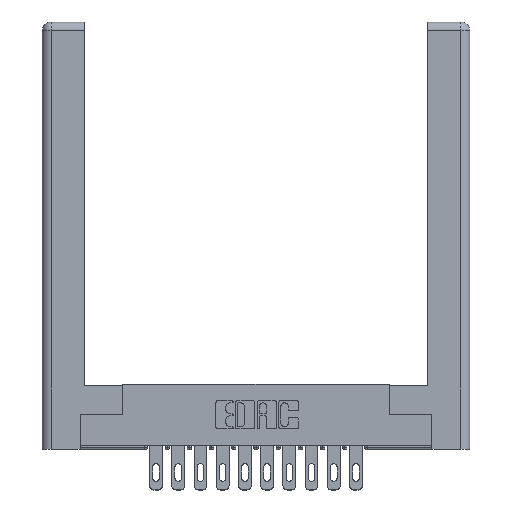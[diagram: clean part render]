
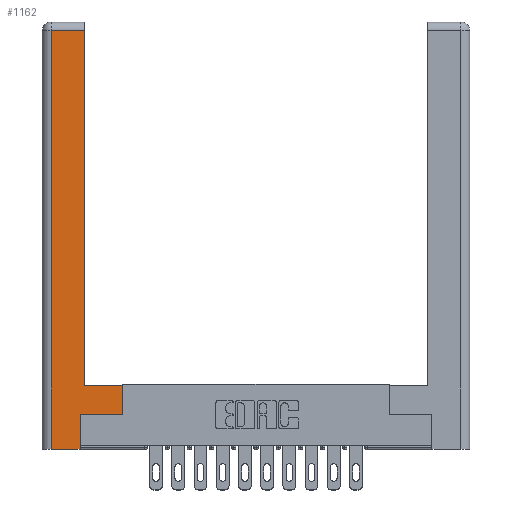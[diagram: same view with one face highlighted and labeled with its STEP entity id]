
A CAD part, top view. The second image highlights one B-rep face of the part: STEP entity #1162.
In plain terms, the highlighted planar face has unit normal (0, 0, 1).
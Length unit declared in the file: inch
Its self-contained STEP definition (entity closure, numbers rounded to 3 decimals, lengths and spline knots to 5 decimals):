
#121 = VERTEX_POINT ( 'NONE', #6297 ) ;
#192 = EDGE_CURVE ( 'NONE', #15788, #4579, #12210, .T. ) ;
#621 = DIRECTION ( 'NONE',  ( 0., 0., -1. ) ) ;
#874 = LINE ( 'NONE', #12211, #16828 ) ;
#901 = EDGE_CURVE ( 'NONE', #14083, #13963, #13010, .T. ) ;
#926 = VECTOR ( 'NONE', #5766, 39.37008 ) ;
#1162 = ADVANCED_FACE ( 'NONE', ( #10686 ), #7216, .F. ) ;
#1360 = EDGE_CURVE ( 'NONE', #4579, #14083, #15285, .T. ) ;
#2516 = LINE ( 'NONE', #7158, #15133 ) ;
#2532 = CARTESIAN_POINT ( 'NONE',  ( 0.0615, 0., 0. ) ) ;
#3534 = ORIENTED_EDGE ( 'NONE', *, *, #13781, .T. ) ;
#3814 = CARTESIAN_POINT ( 'NONE',  ( 0.265, 0.245, 0. ) ) ;
#3892 = DIRECTION ( 'NONE',  ( 0., -1., 0. ) ) ;
#4003 = LINE ( 'NONE', #13521, #13904 ) ;
#4579 = VERTEX_POINT ( 'NONE', #13706 ) ;
#5587 = ORIENTED_EDGE ( 'NONE', *, *, #8239, .T. ) ;
#5591 = CARTESIAN_POINT ( 'NONE',  ( 0.565, 0.245, 0. ) ) ;
#5766 = DIRECTION ( 'NONE',  ( 1., 0., 0. ) ) ;
#5861 = DIRECTION ( 'NONE',  ( 1., 0., 0. ) ) ;
#5960 = ORIENTED_EDGE ( 'NONE', *, *, #901, .T. ) ;
#6172 = DIRECTION ( 'NONE',  ( -1., 0., 0. ) ) ;
#6297 = CARTESIAN_POINT ( 'NONE',  ( 0.295, 0.45, 0. ) ) ;
#6463 = ORIENTED_EDGE ( 'NONE', *, *, #192, .T. ) ;
#6535 = CARTESIAN_POINT ( 'NONE',  ( 0.265, 0., 0. ) ) ;
#6667 = VERTEX_POINT ( 'NONE', #9449 ) ;
#7158 = CARTESIAN_POINT ( 'NONE',  ( 0.565, 0.45, 0. ) ) ;
#7216 = PLANE ( 'NONE',  #12391 ) ;
#7611 = EDGE_CURVE ( 'NONE', #121, #11148, #4003, .T. ) ;
#8143 = ORIENTED_EDGE ( 'NONE', *, *, #12999, .T. ) ;
#8239 = EDGE_CURVE ( 'NONE', #6667, #121, #14307, .T. ) ;
#8377 = VERTEX_POINT ( 'NONE', #13643 ) ;
#8545 = CARTESIAN_POINT ( 'NONE',  ( 0.265, 0., 0. ) ) ;
#8658 = DIRECTION ( 'NONE',  ( -1., 0., 0. ) ) ;
#9424 = VECTOR ( 'NONE', #16846, 39.37008 ) ;
#9449 = CARTESIAN_POINT ( 'NONE',  ( 0.565, 0.45, 0. ) ) ;
#9746 = CARTESIAN_POINT ( 'NONE',  ( 0.0615, 2.94, 0. ) ) ;
#10246 = EDGE_LOOP ( 'NONE', ( #14707, #8143, #6463, #16505, #5960, #17355, #3534, #5587 ) ) ;
#10686 = FACE_OUTER_BOUND ( 'NONE', #10246, .T. ) ;
#11148 = VERTEX_POINT ( 'NONE', #11931 ) ;
#11931 = CARTESIAN_POINT ( 'NONE',  ( 0.295, 2.94, 0. ) ) ;
#12198 = VECTOR ( 'NONE', #6172, 39.37008 ) ;
#12210 = LINE ( 'NONE', #2532, #16605 ) ;
#12211 = CARTESIAN_POINT ( 'NONE',  ( 0.0615, 2.94, 0. ) ) ;
#12391 = AXIS2_PLACEMENT_3D ( 'NONE', #16701, #621, #8658 ) ;
#12459 = LINE ( 'NONE', #5591, #926 ) ;
#12884 = CARTESIAN_POINT ( 'NONE',  ( 0.295, 0.45, 0. ) ) ;
#12999 = EDGE_CURVE ( 'NONE', #11148, #15788, #874, .T. ) ;
#13010 = LINE ( 'NONE', #15267, #9424 ) ;
#13521 = CARTESIAN_POINT ( 'NONE',  ( 0.295, 3., 0. ) ) ;
#13643 = CARTESIAN_POINT ( 'NONE',  ( 0.565, 0.245, 0. ) ) ;
#13706 = CARTESIAN_POINT ( 'NONE',  ( 0.0615, 0., 0. ) ) ;
#13781 = EDGE_CURVE ( 'NONE', #8377, #6667, #2516, .T. ) ;
#13904 = VECTOR ( 'NONE', #14708, 39.37008 ) ;
#13963 = VERTEX_POINT ( 'NONE', #3814 ) ;
#14083 = VERTEX_POINT ( 'NONE', #6535 ) ;
#14307 = LINE ( 'NONE', #12884, #12198 ) ;
#14460 = VECTOR ( 'NONE', #5861, 39.37008 ) ;
#14707 = ORIENTED_EDGE ( 'NONE', *, *, #7611, .T. ) ;
#14708 = DIRECTION ( 'NONE',  ( 0., 1., 0. ) ) ;
#15133 = VECTOR ( 'NONE', #16576, 39.37008 ) ;
#15267 = CARTESIAN_POINT ( 'NONE',  ( 0.265, 0.245, 0. ) ) ;
#15285 = LINE ( 'NONE', #8545, #14460 ) ;
#15788 = VERTEX_POINT ( 'NONE', #9746 ) ;
#16233 = DIRECTION ( 'NONE',  ( -1., 0., 0. ) ) ;
#16505 = ORIENTED_EDGE ( 'NONE', *, *, #1360, .T. ) ;
#16576 = DIRECTION ( 'NONE',  ( 0., 1., 0. ) ) ;
#16605 = VECTOR ( 'NONE', #3892, 39.37008 ) ;
#16701 = CARTESIAN_POINT ( 'NONE',  ( 0., 0., 0. ) ) ;
#16828 = VECTOR ( 'NONE', #16233, 39.37008 ) ;
#16846 = DIRECTION ( 'NONE',  ( 0., 1., 0. ) ) ;
#17077 = EDGE_CURVE ( 'NONE', #13963, #8377, #12459, .T. ) ;
#17355 = ORIENTED_EDGE ( 'NONE', *, *, #17077, .T. ) ;
